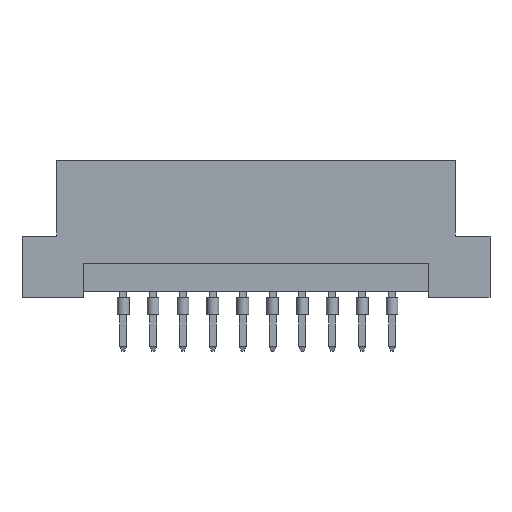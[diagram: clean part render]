
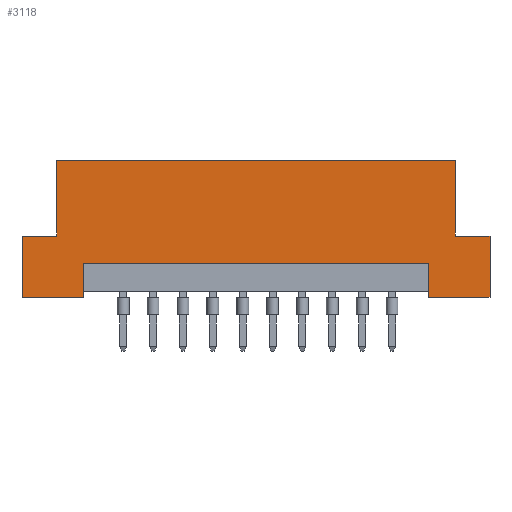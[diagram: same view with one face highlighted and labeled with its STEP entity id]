
A CAD part, front view. The second image highlights one B-rep face of the part: STEP entity #3118.
In plain terms, the highlighted planar face has unit normal (0, -1, 0).
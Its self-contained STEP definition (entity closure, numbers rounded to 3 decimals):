
#164 = LINE ( 'NONE', #2373, #410 ) ;
#232 = LINE ( 'NONE', #1840, #5261 ) ;
#410 = VECTOR ( 'NONE', #4599, 1000. ) ;
#428 = EDGE_CURVE ( 'NONE', #2114, #4659, #2411, .T. ) ;
#451 = VECTOR ( 'NONE', #6332, 1000. ) ;
#563 = EDGE_CURVE ( 'NONE', #4968, #2729, #930, .T. ) ;
#582 = CARTESIAN_POINT ( 'NONE',  ( -19.9, 0., 0. ) ) ;
#790 = CARTESIAN_POINT ( 'NONE',  ( -16.94, 0., 5.2 ) ) ;
#830 = EDGE_CURVE ( 'NONE', #4664, #4714, #232, .T. ) ;
#855 = VECTOR ( 'NONE', #2786, 1000. ) ;
#892 = CARTESIAN_POINT ( 'NONE',  ( 14.69, 0., 0.5 ) ) ;
#921 = DIRECTION ( 'NONE',  ( 0., 0., 1. ) ) ;
#930 = LINE ( 'NONE', #7113, #1542 ) ;
#950 = EDGE_CURVE ( 'NONE', #2812, #5061, #3732, .T. ) ;
#963 = DIRECTION ( 'NONE',  ( -1., 0., 0. ) ) ;
#988 = ORIENTED_EDGE ( 'NONE', *, *, #6305, .F. ) ;
#1439 = ORIENTED_EDGE ( 'NONE', *, *, #5440, .F. ) ;
#1542 = VECTOR ( 'NONE', #963, 1000. ) ;
#1634 = DIRECTION ( 'NONE',  ( 0., 0., -1. ) ) ;
#1669 = VECTOR ( 'NONE', #5886, 1000. ) ;
#1840 = CARTESIAN_POINT ( 'NONE',  ( -16.94, 0., 5.2 ) ) ;
#1913 = CARTESIAN_POINT ( 'NONE',  ( 16.94, 0., 5.2 ) ) ;
#1971 = VECTOR ( 'NONE', #2764, 1000. ) ;
#1980 = ORIENTED_EDGE ( 'NONE', *, *, #6822, .F. ) ;
#1992 = AXIS2_PLACEMENT_3D ( 'NONE', #4364, #4328, #6580 ) ;
#2002 = VECTOR ( 'NONE', #2754, 1000. ) ;
#2103 = VERTEX_POINT ( 'NONE', #6002 ) ;
#2109 = FACE_OUTER_BOUND ( 'NONE', #5764, .T. ) ;
#2114 = VERTEX_POINT ( 'NONE', #7090 ) ;
#2218 = CARTESIAN_POINT ( 'NONE',  ( 19.9, 0., 5.2 ) ) ;
#2324 = EDGE_CURVE ( 'NONE', #4659, #6340, #164, .T. ) ;
#2373 = CARTESIAN_POINT ( 'NONE',  ( -14.69, 0., 0.5 ) ) ;
#2398 = VERTEX_POINT ( 'NONE', #3658 ) ;
#2411 = LINE ( 'NONE', #3668, #1669 ) ;
#2541 = ORIENTED_EDGE ( 'NONE', *, *, #2324, .F. ) ;
#2729 = VERTEX_POINT ( 'NONE', #6775 ) ;
#2754 = DIRECTION ( 'NONE',  ( 1., 0., 0. ) ) ;
#2764 = DIRECTION ( 'NONE',  ( 1., 0., 0. ) ) ;
#2775 = LINE ( 'NONE', #5042, #4974 ) ;
#2786 = DIRECTION ( 'NONE',  ( -1., 0., 0. ) ) ;
#2812 = VERTEX_POINT ( 'NONE', #6317 ) ;
#3010 = ORIENTED_EDGE ( 'NONE', *, *, #428, .F. ) ;
#3118 = ADVANCED_FACE ( 'NONE', ( #2109 ), #7172, .F. ) ;
#3417 = ORIENTED_EDGE ( 'NONE', *, *, #563, .F. ) ;
#3618 = LINE ( 'NONE', #892, #451 ) ;
#3658 = CARTESIAN_POINT ( 'NONE',  ( -19.9, 0., 5.2 ) ) ;
#3668 = CARTESIAN_POINT ( 'NONE',  ( 14.69, 0., 2.9 ) ) ;
#3732 = LINE ( 'NONE', #1913, #4798 ) ;
#3896 = LINE ( 'NONE', #582, #855 ) ;
#3913 = EDGE_CURVE ( 'NONE', #2812, #2103, #5459, .T. ) ;
#3941 = DIRECTION ( 'NONE',  ( 1., 0., 0. ) ) ;
#3957 = DIRECTION ( 'NONE',  ( 0., 0., 1. ) ) ;
#3988 = EDGE_CURVE ( 'NONE', #2103, #4968, #5421, .T. ) ;
#3998 = CARTESIAN_POINT ( 'NONE',  ( -14.69, 0., 0. ) ) ;
#4328 = DIRECTION ( 'NONE',  ( 0., 1., 0. ) ) ;
#4364 = CARTESIAN_POINT ( 'NONE',  ( -19.9, 0., 11.6 ) ) ;
#4365 = CARTESIAN_POINT ( 'NONE',  ( 19.9, 0., 0. ) ) ;
#4564 = EDGE_CURVE ( 'NONE', #6340, #6518, #3896, .T. ) ;
#4599 = DIRECTION ( 'NONE',  ( 0., 0., -1. ) ) ;
#4659 = VERTEX_POINT ( 'NONE', #5747 ) ;
#4664 = VERTEX_POINT ( 'NONE', #790 ) ;
#4714 = VERTEX_POINT ( 'NONE', #6530 ) ;
#4798 = VECTOR ( 'NONE', #921, 1000. ) ;
#4816 = ORIENTED_EDGE ( 'NONE', *, *, #830, .F. ) ;
#4851 = ORIENTED_EDGE ( 'NONE', *, *, #950, .T. ) ;
#4882 = ORIENTED_EDGE ( 'NONE', *, *, #6412, .T. ) ;
#4968 = VERTEX_POINT ( 'NONE', #5765 ) ;
#4974 = VECTOR ( 'NONE', #6754, 1000. ) ;
#5042 = CARTESIAN_POINT ( 'NONE',  ( -19.9, 0., 0. ) ) ;
#5061 = VERTEX_POINT ( 'NONE', #5178 ) ;
#5066 = LINE ( 'NONE', #6243, #6765 ) ;
#5178 = CARTESIAN_POINT ( 'NONE',  ( 16.94, 0., 11.6 ) ) ;
#5261 = VECTOR ( 'NONE', #3957, 1000. ) ;
#5369 = VECTOR ( 'NONE', #1634, 1000. ) ;
#5421 = LINE ( 'NONE', #4365, #5369 ) ;
#5440 = EDGE_CURVE ( 'NONE', #4714, #5061, #5066, .T. ) ;
#5459 = LINE ( 'NONE', #2218, #2002 ) ;
#5657 = LINE ( 'NONE', #6253, #1971 ) ;
#5747 = CARTESIAN_POINT ( 'NONE',  ( -14.69, 0., 2.9 ) ) ;
#5764 = EDGE_LOOP ( 'NONE', ( #3010, #4882, #3417, #6415, #6038, #4851, #1439, #4816, #1980, #988, #6047, #2541 ) ) ;
#5765 = CARTESIAN_POINT ( 'NONE',  ( 19.9, 0., 0. ) ) ;
#5886 = DIRECTION ( 'NONE',  ( -1., 0., 0. ) ) ;
#6002 = CARTESIAN_POINT ( 'NONE',  ( 19.9, 0., 5.2 ) ) ;
#6038 = ORIENTED_EDGE ( 'NONE', *, *, #3913, .F. ) ;
#6047 = ORIENTED_EDGE ( 'NONE', *, *, #4564, .F. ) ;
#6243 = CARTESIAN_POINT ( 'NONE',  ( -19.9, 0., 11.6 ) ) ;
#6253 = CARTESIAN_POINT ( 'NONE',  ( -19.9, 0., 5.2 ) ) ;
#6305 = EDGE_CURVE ( 'NONE', #6518, #2398, #2775, .T. ) ;
#6317 = CARTESIAN_POINT ( 'NONE',  ( 16.94, 0., 5.2 ) ) ;
#6332 = DIRECTION ( 'NONE',  ( 0., 0., -1. ) ) ;
#6340 = VERTEX_POINT ( 'NONE', #3998 ) ;
#6369 = CARTESIAN_POINT ( 'NONE',  ( -19.9, 0., 0. ) ) ;
#6412 = EDGE_CURVE ( 'NONE', #2114, #2729, #3618, .T. ) ;
#6415 = ORIENTED_EDGE ( 'NONE', *, *, #3988, .F. ) ;
#6518 = VERTEX_POINT ( 'NONE', #6369 ) ;
#6530 = CARTESIAN_POINT ( 'NONE',  ( -16.94, 0., 11.6 ) ) ;
#6580 = DIRECTION ( 'NONE',  ( 0., 0., 1. ) ) ;
#6754 = DIRECTION ( 'NONE',  ( 0., 0., 1. ) ) ;
#6765 = VECTOR ( 'NONE', #3941, 1000. ) ;
#6775 = CARTESIAN_POINT ( 'NONE',  ( 14.69, 0., 0. ) ) ;
#6822 = EDGE_CURVE ( 'NONE', #2398, #4664, #5657, .T. ) ;
#7090 = CARTESIAN_POINT ( 'NONE',  ( 14.69, 0., 2.9 ) ) ;
#7113 = CARTESIAN_POINT ( 'NONE',  ( -19.9, 0., 0. ) ) ;
#7172 = PLANE ( 'NONE',  #1992 ) ;
